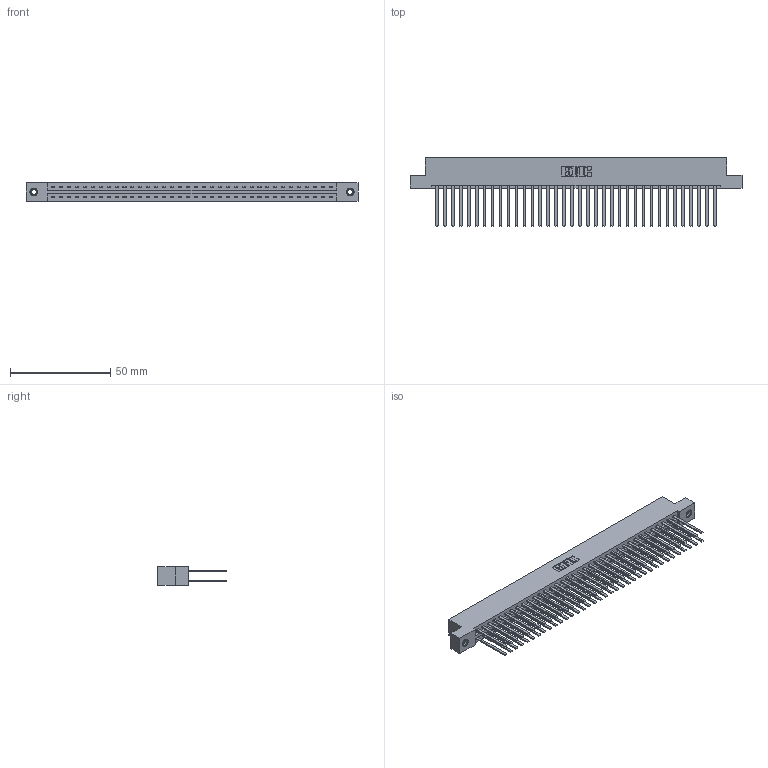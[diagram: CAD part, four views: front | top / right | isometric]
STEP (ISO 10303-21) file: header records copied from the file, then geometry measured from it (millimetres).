
FILE_DESCRIPTION (( 'STEP AP203' ), '1' );
FILE_NAME ('387-072-544-207.STEP', '2018-09-22T18:30:44', ( '' ), ( '' ), 'SwSTEP 2.0', 'SolidWorks 2016', '' );
FILE_SCHEMA (( 'CONFIG_CONTROL_DESIGN' ));
Length unit declared in the file: inch
Products named in the file (4): 337 Part_Flush Mounting Lugs - 0.156 Dia-TI; 345-292-001_345-293-144; 345-250-001_345-250-005-103; 387-072-544-207
Assembly tree (75 placements, depth 2):
  387-072-544-207
    337 Part_Flush Mounting Lugs - 0.156 Dia-TI
    345-292-001_345-293-144  x72
    345-250-001_345-250-005-103  x2
Bounding box: 165.66 x 34.3 x 9.4 mm (x, y, z)
Volume: 18374.4 mm3; surface area: 24047.1 mm2
Topology: 75 solids, 75 shells, 3630 faces, 10743 edges, 7058 vertices
Faces by surface type: plane 2550, cylinder 1064, cone 12, torus 4
Entity records: 29690 total; most frequent: CARTESIAN_POINT 4985, ORIENTED_EDGE 4914, DIRECTION 4279, EDGE_CURVE 2457, LINE 2313, VECTOR 2313, VERTEX_POINT 1632, AXIS2_PLACEMENT_3D 983
